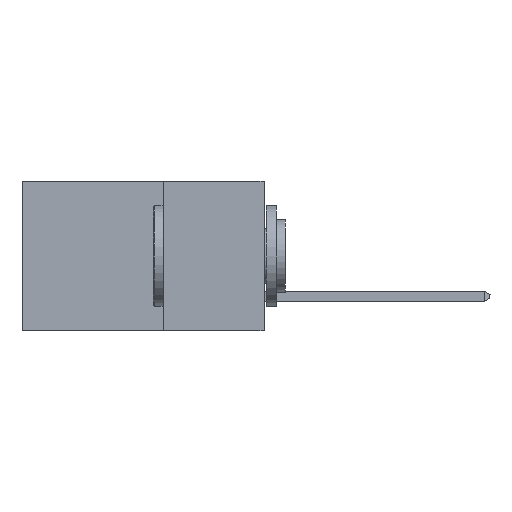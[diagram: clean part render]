
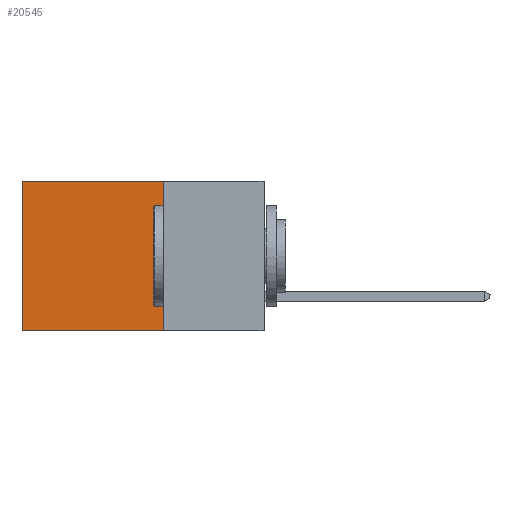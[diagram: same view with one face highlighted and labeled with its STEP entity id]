
A CAD part, left-side view. The second image highlights one B-rep face of the part: STEP entity #20545.
In plain terms, the highlighted planar face has unit normal (-1, 0, 0).
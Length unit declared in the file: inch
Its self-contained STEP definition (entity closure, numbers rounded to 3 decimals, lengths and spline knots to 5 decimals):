
#426 = CARTESIAN_POINT ( 'NONE',  ( 0.2615, 0.6, -0.37 ) ) ;
#557 = EDGE_CURVE ( 'NONE', #14329, #15728, #17355, .T. ) ;
#771 = LINE ( 'NONE', #426, #10316 ) ;
#1559 = CARTESIAN_POINT ( 'NONE',  ( 0.2615, 0.6, 0. ) ) ;
#1893 = EDGE_CURVE ( 'NONE', #15853, #15027, #771, .T. ) ;
#1929 = VECTOR ( 'NONE', #13797, 39.37008 ) ;
#2567 = CARTESIAN_POINT ( 'NONE',  ( 0.2615, 0.25, 0. ) ) ;
#3064 = CARTESIAN_POINT ( 'NONE',  ( 0.2615, 0.6, -0.37 ) ) ;
#5089 = PLANE ( 'NONE',  #18338 ) ;
#5173 = CARTESIAN_POINT ( 'NONE',  ( 0.2615, 0.25, -0.37 ) ) ;
#7230 = DIRECTION ( 'NONE',  ( 0., 1., 0. ) ) ;
#7545 = VECTOR ( 'NONE', #18211, 39.37008 ) ;
#8518 = EDGE_LOOP ( 'NONE', ( #10986, #23001, #8695, #21568 ) ) ;
#8695 = ORIENTED_EDGE ( 'NONE', *, *, #557, .F. ) ;
#8863 = DIRECTION ( 'NONE',  ( 0., 0., -1. ) ) ;
#10316 = VECTOR ( 'NONE', #23567, 39.37008 ) ;
#10761 = CARTESIAN_POINT ( 'NONE',  ( 0.2615, 0.25, 0. ) ) ;
#10986 = ORIENTED_EDGE ( 'NONE', *, *, #1893, .T. ) ;
#12377 = VECTOR ( 'NONE', #7230, 39.37008 ) ;
#13797 = DIRECTION ( 'NONE',  ( 0., 1., 0. ) ) ;
#14329 = VERTEX_POINT ( 'NONE', #10761 ) ;
#14337 = CARTESIAN_POINT ( 'NONE',  ( 0.2615, 0.25, -0.37 ) ) ;
#15027 = VERTEX_POINT ( 'NONE', #3064 ) ;
#15686 = FACE_OUTER_BOUND ( 'NONE', #8518, .T. ) ;
#15728 = VERTEX_POINT ( 'NONE', #14337 ) ;
#15853 = VERTEX_POINT ( 'NONE', #1559 ) ;
#16620 = CARTESIAN_POINT ( 'NONE',  ( 0.2615, 0.25, -0.37 ) ) ;
#16851 = LINE ( 'NONE', #2567, #1929 ) ;
#17222 = LINE ( 'NONE', #5173, #12377 ) ;
#17355 = LINE ( 'NONE', #16620, #7545 ) ;
#18046 = CARTESIAN_POINT ( 'NONE',  ( 0.2615, 0.25, -0.37 ) ) ;
#18211 = DIRECTION ( 'NONE',  ( 0., 0., -1. ) ) ;
#18338 = AXIS2_PLACEMENT_3D ( 'NONE', #18046, #19821, #8863 ) ;
#19584 = EDGE_CURVE ( 'NONE', #14329, #15853, #16851, .T. ) ;
#19821 = DIRECTION ( 'NONE',  ( 1., 0., 0. ) ) ;
#20545 = ADVANCED_FACE ( 'NONE', ( #15686 ), #5089, .F. ) ;
#21568 = ORIENTED_EDGE ( 'NONE', *, *, #19584, .T. ) ;
#23001 = ORIENTED_EDGE ( 'NONE', *, *, #23784, .F. ) ;
#23567 = DIRECTION ( 'NONE',  ( 0., 0., -1. ) ) ;
#23784 = EDGE_CURVE ( 'NONE', #15728, #15027, #17222, .T. ) ;
